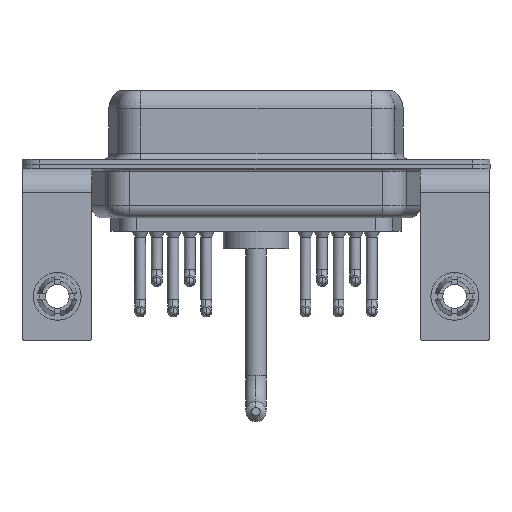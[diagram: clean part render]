
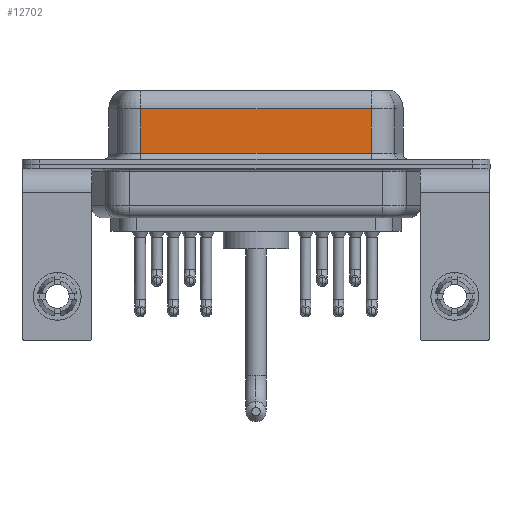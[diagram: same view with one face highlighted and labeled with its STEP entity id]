
A CAD part, front view. The second image highlights one B-rep face of the part: STEP entity #12702.
In plain terms, the highlighted planar face has unit normal (0, -1, 0).
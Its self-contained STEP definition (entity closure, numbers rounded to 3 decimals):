
#456 = DIRECTION ( 'NONE',  ( -1., 0., 0. ) ) ;
#551 = LINE ( 'NONE', #13579, #10377 ) ;
#801 = EDGE_CURVE ( 'NONE', #18785, #17991, #14995, .T. ) ;
#2508 = VERTEX_POINT ( 'NONE', #8343 ) ;
#4358 = ORIENTED_EDGE ( 'NONE', *, *, #17180, .T. ) ;
#4823 = AXIS2_PLACEMENT_3D ( 'NONE', #12462, #7885, #17472 ) ;
#4932 = VERTEX_POINT ( 'NONE', #9696 ) ;
#5492 = VECTOR ( 'NONE', #18292, 1000. ) ;
#6268 = PLANE ( 'NONE',  #4823 ) ;
#7072 = VECTOR ( 'NONE', #11289, 1000. ) ;
#7080 = CARTESIAN_POINT ( 'NONE',  ( 26.287, -3.95, 0.9 ) ) ;
#7670 = FACE_OUTER_BOUND ( 'NONE', #8657, .T. ) ;
#7885 = DIRECTION ( 'NONE',  ( 0., 1., 0. ) ) ;
#8343 = CARTESIAN_POINT ( 'NONE',  ( 26.287, -3.95, 4.65 ) ) ;
#8657 = EDGE_LOOP ( 'NONE', ( #11693, #14939, #4358, #20807 ) ) ;
#9582 = LINE ( 'NONE', #14272, #15428 ) ;
#9696 = CARTESIAN_POINT ( 'NONE',  ( 7.013, -3.95, 4.65 ) ) ;
#10377 = VECTOR ( 'NONE', #456, 1000. ) ;
#10968 = LINE ( 'NONE', #19177, #7072 ) ;
#11289 = DIRECTION ( 'NONE',  ( 0., 0., -1. ) ) ;
#11693 = ORIENTED_EDGE ( 'NONE', *, *, #14123, .F. ) ;
#12462 = CARTESIAN_POINT ( 'NONE',  ( 26.287, -3.95, 6.4 ) ) ;
#12702 = ADVANCED_FACE ( 'NONE', ( #7670 ), #6268, .F. ) ;
#13579 = CARTESIAN_POINT ( 'NONE',  ( 26.287, -3.95, 4.65 ) ) ;
#14123 = EDGE_CURVE ( 'NONE', #2508, #17991, #9582, .T. ) ;
#14272 = CARTESIAN_POINT ( 'NONE',  ( 26.287, -3.95, 6.4 ) ) ;
#14788 = CARTESIAN_POINT ( 'NONE',  ( 26.287, -3.95, 0.9 ) ) ;
#14939 = ORIENTED_EDGE ( 'NONE', *, *, #15309, .T. ) ;
#14995 = LINE ( 'NONE', #14788, #5492 ) ;
#15309 = EDGE_CURVE ( 'NONE', #2508, #4932, #551, .T. ) ;
#15428 = VECTOR ( 'NONE', #20767, 1000. ) ;
#16255 = CARTESIAN_POINT ( 'NONE',  ( 7.013, -3.95, 0.9 ) ) ;
#17180 = EDGE_CURVE ( 'NONE', #4932, #18785, #10968, .T. ) ;
#17472 = DIRECTION ( 'NONE',  ( 0., 0., 1. ) ) ;
#17991 = VERTEX_POINT ( 'NONE', #7080 ) ;
#18292 = DIRECTION ( 'NONE',  ( 1., 0., 0. ) ) ;
#18785 = VERTEX_POINT ( 'NONE', #16255 ) ;
#19177 = CARTESIAN_POINT ( 'NONE',  ( 7.013, -3.95, 6.4 ) ) ;
#20767 = DIRECTION ( 'NONE',  ( 0., 0., -1. ) ) ;
#20807 = ORIENTED_EDGE ( 'NONE', *, *, #801, .T. ) ;
